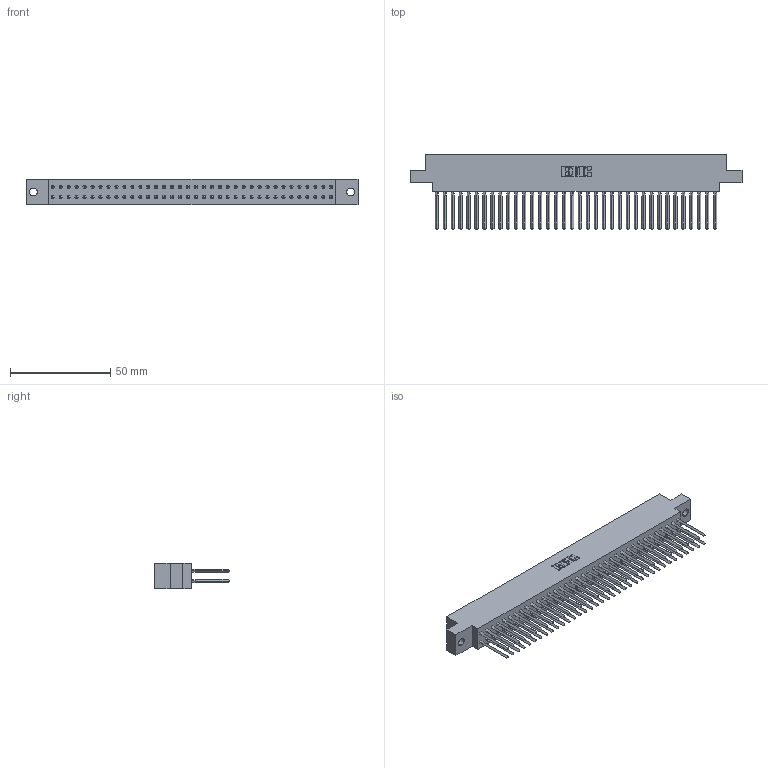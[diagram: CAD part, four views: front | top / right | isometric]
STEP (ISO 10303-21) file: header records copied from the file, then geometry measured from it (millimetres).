
FILE_DESCRIPTION (( 'STEP AP203' ), '1' );
FILE_NAME ('317-072-540-804.STEP', '2020-02-28T07:24:43', ( '' ), ( '' ), 'SwSTEP 2.0', 'SolidWorks 2016', '' );
FILE_SCHEMA (( 'CONFIG_CONTROL_DESIGN' ));
Length unit declared in the file: inch
Products named in the file (3): 317 Part_.156 Dia - TH; 317-072-540-804; 317-290-001_540
Assembly tree (73 placements, depth 2):
  317-072-540-804
    317 Part_.156 Dia - TH
    317-290-001_540  x72
Bounding box: 165.35 x 37.34 x 12.7 mm (x, y, z)
Volume: 27460.8 mm3; surface area: 40540.1 mm2
Topology: 73 solids, 73 shells, 6510 faces, 18059 edges, 11630 vertices
Faces by surface type: plane 5314, cylinder 908, bspline 288
Entity records: 52878 total; most frequent: CARTESIAN_POINT 9639, ORIENTED_EDGE 9138, DIRECTION 7623, EDGE_CURVE 4569, LINE 4313, VECTOR 4313, VERTEX_POINT 3039, AXIS2_PLACEMENT_3D 1655
